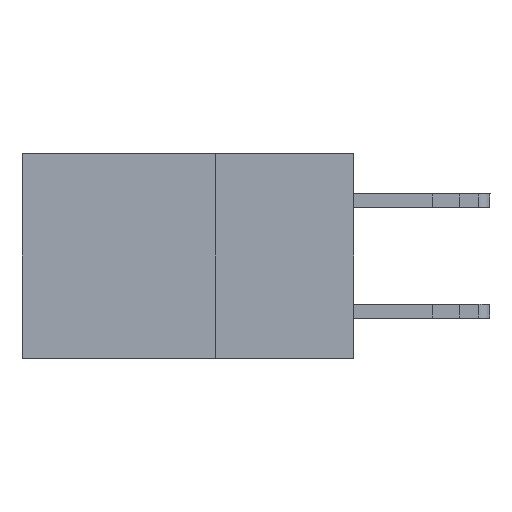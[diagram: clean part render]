
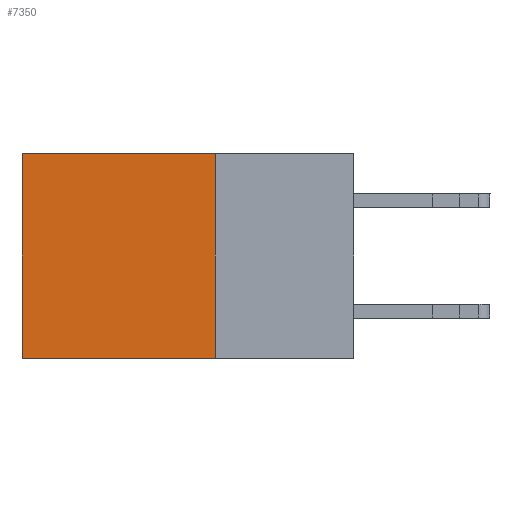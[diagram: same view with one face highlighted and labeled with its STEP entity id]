
A CAD part, left-side view. The second image highlights one B-rep face of the part: STEP entity #7350.
In plain terms, the highlighted planar face has unit normal (-1, 0, 0).
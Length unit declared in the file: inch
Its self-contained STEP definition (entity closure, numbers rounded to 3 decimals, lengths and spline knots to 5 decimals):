
#165 = CARTESIAN_POINT ( 'NONE',  ( 0.2875, 0.6, -0.37 ) ) ;
#364 = CARTESIAN_POINT ( 'NONE',  ( 0.2875, 0.25, 0. ) ) ;
#665 = LINE ( 'NONE', #3479, #19622 ) ;
#1295 = FACE_OUTER_BOUND ( 'NONE', #15767, .T. ) ;
#2004 = LINE ( 'NONE', #23228, #21545 ) ;
#3070 = ORIENTED_EDGE ( 'NONE', *, *, #11009, .T. ) ;
#3479 = CARTESIAN_POINT ( 'NONE',  ( 0.2875, 0.25, -0.37 ) ) ;
#4216 = CARTESIAN_POINT ( 'NONE',  ( 0.2875, 0.6, 0. ) ) ;
#4265 = EDGE_CURVE ( 'NONE', #8465, #7174, #8039, .T. ) ;
#5021 = VERTEX_POINT ( 'NONE', #165 ) ;
#6802 = CARTESIAN_POINT ( 'NONE',  ( 0.2875, 0.25, 0. ) ) ;
#7097 = EDGE_CURVE ( 'NONE', #11021, #5021, #665, .T. ) ;
#7174 = VERTEX_POINT ( 'NONE', #8838 ) ;
#7350 = ADVANCED_FACE ( 'NONE', ( #1295 ), #18999, .F. ) ;
#8039 = LINE ( 'NONE', #6802, #8919 ) ;
#8465 = VERTEX_POINT ( 'NONE', #364 ) ;
#8584 = DIRECTION ( 'NONE',  ( 0., 0., -1. ) ) ;
#8838 = CARTESIAN_POINT ( 'NONE',  ( 0.2875, 0.6, 0. ) ) ;
#8875 = DIRECTION ( 'NONE',  ( 0., 1., 0. ) ) ;
#8919 = VECTOR ( 'NONE', #8875, 39.37008 ) ;
#9501 = EDGE_CURVE ( 'NONE', #8465, #11021, #2004, .T. ) ;
#10846 = DIRECTION ( 'NONE',  ( 0., 1., 0. ) ) ;
#11009 = EDGE_CURVE ( 'NONE', #7174, #5021, #16011, .T. ) ;
#11021 = VERTEX_POINT ( 'NONE', #22294 ) ;
#15767 = EDGE_LOOP ( 'NONE', ( #3070, #16816, #17765, #20677 ) ) ;
#16011 = LINE ( 'NONE', #4216, #22203 ) ;
#16816 = ORIENTED_EDGE ( 'NONE', *, *, #7097, .F. ) ;
#17221 = DIRECTION ( 'NONE',  ( 0., 0., -1. ) ) ;
#17646 = DIRECTION ( 'NONE',  ( 1., 0., 0. ) ) ;
#17765 = ORIENTED_EDGE ( 'NONE', *, *, #9501, .F. ) ;
#18656 = AXIS2_PLACEMENT_3D ( 'NONE', #22940, #17646, #23694 ) ;
#18999 = PLANE ( 'NONE',  #18656 ) ;
#19622 = VECTOR ( 'NONE', #10846, 39.37008 ) ;
#20677 = ORIENTED_EDGE ( 'NONE', *, *, #4265, .T. ) ;
#21545 = VECTOR ( 'NONE', #8584, 39.37008 ) ;
#22203 = VECTOR ( 'NONE', #17221, 39.37008 ) ;
#22294 = CARTESIAN_POINT ( 'NONE',  ( 0.2875, 0.25, -0.37 ) ) ;
#22940 = CARTESIAN_POINT ( 'NONE',  ( 0.2875, 0.25, 0. ) ) ;
#23228 = CARTESIAN_POINT ( 'NONE',  ( 0.2875, 0.25, 0. ) ) ;
#23694 = DIRECTION ( 'NONE',  ( 0., 0., -1. ) ) ;
